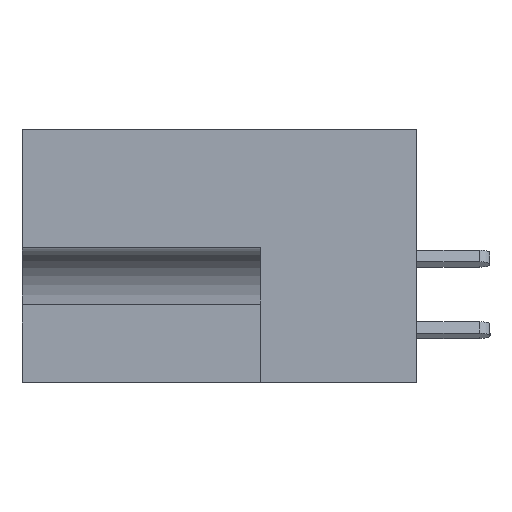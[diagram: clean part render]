
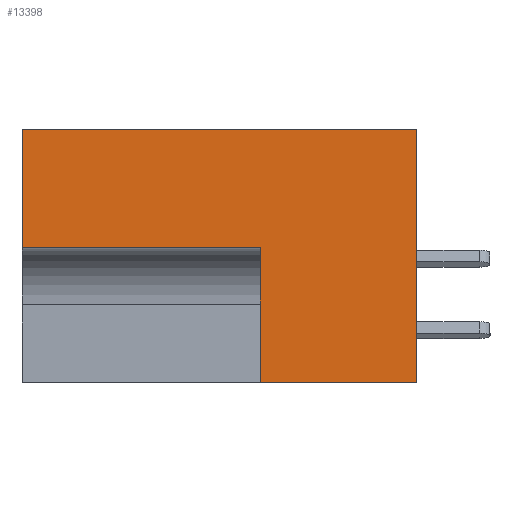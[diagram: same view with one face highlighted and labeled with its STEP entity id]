
A CAD part, left-side view. The second image highlights one B-rep face of the part: STEP entity #13398.
In plain terms, the highlighted planar face has unit normal (-1, 0, 0).
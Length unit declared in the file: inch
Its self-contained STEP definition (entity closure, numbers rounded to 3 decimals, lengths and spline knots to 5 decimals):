
#1488 = EDGE_CURVE ( 'NONE', #10859, #12927, #12653, .T. ) ;
#2258 = ORIENTED_EDGE ( 'NONE', *, *, #14318, .T. ) ;
#2638 = DIRECTION ( 'NONE',  ( 0., 0., 1. ) ) ;
#2803 = CARTESIAN_POINT ( 'NONE',  ( 0., 0.453, 0. ) ) ;
#2934 = EDGE_LOOP ( 'NONE', ( #14141, #14630, #8881, #8250, #2258, #15144 ) ) ;
#3586 = AXIS2_PLACEMENT_3D ( 'NONE', #14309, #19089, #15784 ) ;
#3598 = CARTESIAN_POINT ( 'NONE',  ( 0., 0.328, -0.531 ) ) ;
#3913 = CARTESIAN_POINT ( 'NONE',  ( 0., 0.328, -0.248 ) ) ;
#4368 = EDGE_CURVE ( 'NONE', #14140, #12887, #16784, .T. ) ;
#4578 = DIRECTION ( 'NONE',  ( 0., 1., 0. ) ) ;
#5182 = FACE_OUTER_BOUND ( 'NONE', #2934, .T. ) ;
#5925 = CARTESIAN_POINT ( 'NONE',  ( 0., 0., 0. ) ) ;
#6398 = EDGE_CURVE ( 'NONE', #10859, #14140, #16462, .T. ) ;
#6399 = VECTOR ( 'NONE', #14216, 39.37008 ) ;
#6766 = VECTOR ( 'NONE', #10734, 39.37008 ) ;
#7435 = LINE ( 'NONE', #12416, #18560 ) ;
#7437 = CARTESIAN_POINT ( 'NONE',  ( 0., 0.453, -0.531 ) ) ;
#7867 = DIRECTION ( 'NONE',  ( 0., 0., 1. ) ) ;
#8250 = ORIENTED_EDGE ( 'NONE', *, *, #1488, .T. ) ;
#8881 = ORIENTED_EDGE ( 'NONE', *, *, #6398, .F. ) ;
#9636 = VECTOR ( 'NONE', #10463, 39.37008 ) ;
#10108 = CARTESIAN_POINT ( 'NONE',  ( 0., 0.828, 0. ) ) ;
#10226 = CARTESIAN_POINT ( 'NONE',  ( 0., 0., -0.531 ) ) ;
#10368 = CARTESIAN_POINT ( 'NONE',  ( 0., 0.828, -0.248 ) ) ;
#10463 = DIRECTION ( 'NONE',  ( 0., 0., 1. ) ) ;
#10734 = DIRECTION ( 'NONE',  ( 0., -1., 0. ) ) ;
#10859 = VERTEX_POINT ( 'NONE', #3598 ) ;
#11084 = CARTESIAN_POINT ( 'NONE',  ( 0., 0.328, -0.531 ) ) ;
#12193 = VECTOR ( 'NONE', #7867, 39.37008 ) ;
#12416 = CARTESIAN_POINT ( 'NONE',  ( 0., 0., 0. ) ) ;
#12506 = VECTOR ( 'NONE', #4578, 39.37008 ) ;
#12653 = LINE ( 'NONE', #7437, #6766 ) ;
#12887 = VERTEX_POINT ( 'NONE', #10368 ) ;
#12927 = VERTEX_POINT ( 'NONE', #10226 ) ;
#13063 = VERTEX_POINT ( 'NONE', #5925 ) ;
#13186 = CARTESIAN_POINT ( 'NONE',  ( 0., 0.828, 0. ) ) ;
#13398 = ADVANCED_FACE ( 'NONE', ( #5182 ), #15655, .F. ) ;
#14140 = VERTEX_POINT ( 'NONE', #3913 ) ;
#14141 = ORIENTED_EDGE ( 'NONE', *, *, #20352, .F. ) ;
#14216 = DIRECTION ( 'NONE',  ( 0., -1., 0. ) ) ;
#14309 = CARTESIAN_POINT ( 'NONE',  ( 0., 0.453, 0. ) ) ;
#14318 = EDGE_CURVE ( 'NONE', #12927, #13063, #7435, .T. ) ;
#14553 = LINE ( 'NONE', #2803, #6399 ) ;
#14620 = CARTESIAN_POINT ( 'NONE',  ( 0., 0.328, -0.248 ) ) ;
#14630 = ORIENTED_EDGE ( 'NONE', *, *, #4368, .F. ) ;
#14739 = VERTEX_POINT ( 'NONE', #13186 ) ;
#15144 = ORIENTED_EDGE ( 'NONE', *, *, #18737, .F. ) ;
#15655 = PLANE ( 'NONE',  #3586 ) ;
#15784 = DIRECTION ( 'NONE',  ( 0., 0., -1. ) ) ;
#16462 = LINE ( 'NONE', #11084, #12193 ) ;
#16784 = LINE ( 'NONE', #14620, #12506 ) ;
#18560 = VECTOR ( 'NONE', #2638, 39.37008 ) ;
#18737 = EDGE_CURVE ( 'NONE', #14739, #13063, #14553, .T. ) ;
#19089 = DIRECTION ( 'NONE',  ( 1., 0., 0. ) ) ;
#20352 = EDGE_CURVE ( 'NONE', #12887, #14739, #20993, .T. ) ;
#20993 = LINE ( 'NONE', #10108, #9636 ) ;
